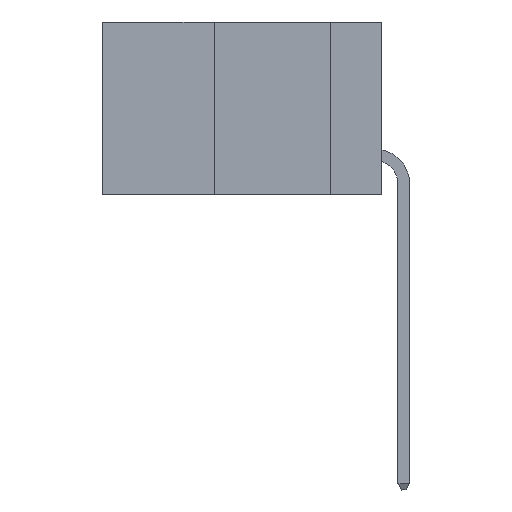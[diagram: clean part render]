
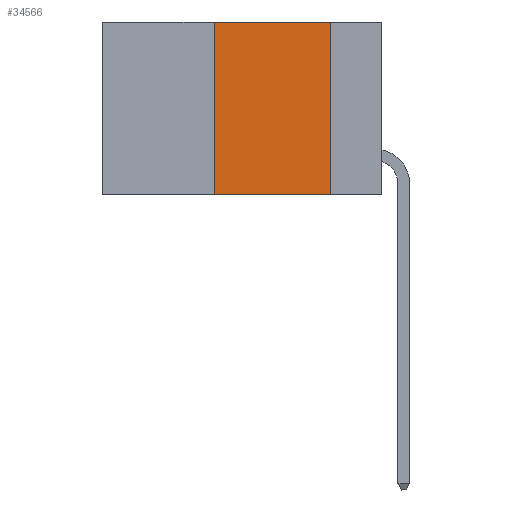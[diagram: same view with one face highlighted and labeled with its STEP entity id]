
A CAD part, left-side view. The second image highlights one B-rep face of the part: STEP entity #34566.
In plain terms, the highlighted planar face has unit normal (-1, 0, 0).
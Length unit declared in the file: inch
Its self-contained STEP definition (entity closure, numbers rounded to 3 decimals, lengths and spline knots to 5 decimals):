
#2691 = LINE ( 'NONE', #23617, #15843 ) ;
#2780 = PLANE ( 'NONE',  #10903 ) ;
#3788 = EDGE_CURVE ( 'NONE', #35673, #13666, #41363, .T. ) ;
#4074 = CARTESIAN_POINT ( 'NONE',  ( 0., 0.11, -0.37 ) ) ;
#4506 = ORIENTED_EDGE ( 'NONE', *, *, #45168, .F. ) ;
#4566 = CARTESIAN_POINT ( 'NONE',  ( 0., 0.11, 0. ) ) ;
#5105 = EDGE_LOOP ( 'NONE', ( #12212, #4506, #33903, #14475 ) ) ;
#6027 = VECTOR ( 'NONE', #47164, 39.37008 ) ;
#9449 = VECTOR ( 'NONE', #40871, 39.37008 ) ;
#9476 = CARTESIAN_POINT ( 'NONE',  ( 0., 0.6, -0.37 ) ) ;
#10903 = AXIS2_PLACEMENT_3D ( 'NONE', #33822, #33131, #30574 ) ;
#11043 = CARTESIAN_POINT ( 'NONE',  ( 0., 0.11, 0. ) ) ;
#12212 = ORIENTED_EDGE ( 'NONE', *, *, #3788, .F. ) ;
#13666 = VERTEX_POINT ( 'NONE', #4074 ) ;
#14475 = ORIENTED_EDGE ( 'NONE', *, *, #19470, .T. ) ;
#15824 = CARTESIAN_POINT ( 'NONE',  ( 0., 0.6, 0. ) ) ;
#15843 = VECTOR ( 'NONE', #27899, 39.37008 ) ;
#19470 = EDGE_CURVE ( 'NONE', #34447, #13666, #41587, .T. ) ;
#23617 = CARTESIAN_POINT ( 'NONE',  ( 0., 0.36, 0. ) ) ;
#24014 = LINE ( 'NONE', #15824, #6027 ) ;
#27899 = DIRECTION ( 'NONE',  ( 0., 0., 1. ) ) ;
#30574 = DIRECTION ( 'NONE',  ( 0., 0., -1. ) ) ;
#32240 = DIRECTION ( 'NONE',  ( 0., -1., 0. ) ) ;
#32247 = CARTESIAN_POINT ( 'NONE',  ( 0., 0.36, 0. ) ) ;
#33131 = DIRECTION ( 'NONE',  ( 1., 0., 0. ) ) ;
#33822 = CARTESIAN_POINT ( 'NONE',  ( 0., 0.6, 0. ) ) ;
#33903 = ORIENTED_EDGE ( 'NONE', *, *, #36714, .F. ) ;
#34447 = VERTEX_POINT ( 'NONE', #37493 ) ;
#34566 = ADVANCED_FACE ( 'NONE', ( #41396 ), #2780, .F. ) ;
#35673 = VERTEX_POINT ( 'NONE', #4566 ) ;
#36714 = EDGE_CURVE ( 'NONE', #34447, #44312, #2691, .T. ) ;
#37493 = CARTESIAN_POINT ( 'NONE',  ( 0., 0.36, -0.37 ) ) ;
#40871 = DIRECTION ( 'NONE',  ( 0., 0., -1. ) ) ;
#41363 = LINE ( 'NONE', #11043, #9449 ) ;
#41396 = FACE_OUTER_BOUND ( 'NONE', #5105, .T. ) ;
#41587 = LINE ( 'NONE', #9476, #46884 ) ;
#44312 = VERTEX_POINT ( 'NONE', #32247 ) ;
#45168 = EDGE_CURVE ( 'NONE', #44312, #35673, #24014, .T. ) ;
#46884 = VECTOR ( 'NONE', #32240, 39.37008 ) ;
#47164 = DIRECTION ( 'NONE',  ( 0., -1., 0. ) ) ;
